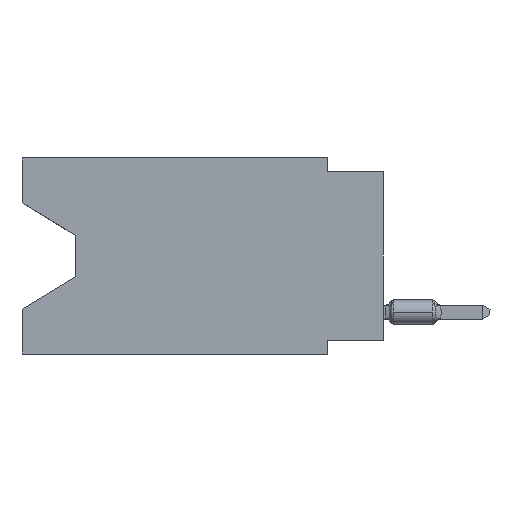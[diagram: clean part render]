
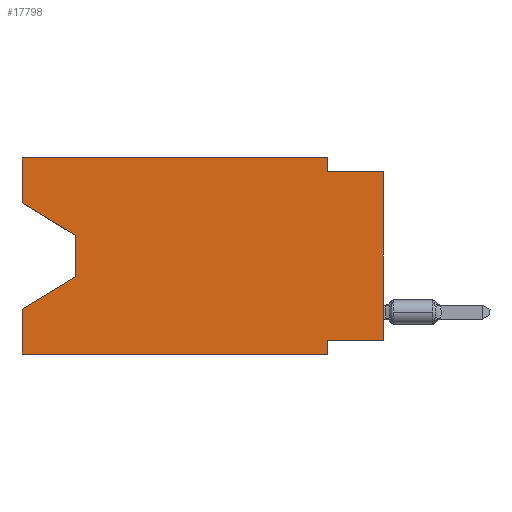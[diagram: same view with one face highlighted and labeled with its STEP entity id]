
A CAD part, left-side view. The second image highlights one B-rep face of the part: STEP entity #17798.
In plain terms, the highlighted planar face has unit normal (-1, 0, 0).
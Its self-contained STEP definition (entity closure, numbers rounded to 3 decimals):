
#36 = ORIENTED_EDGE ( 'NONE', *, *, #11473, .T. ) ;
#167 = VERTEX_POINT ( 'NONE', #1939 ) ;
#609 = DIRECTION ( 'NONE',  ( 0., 0., -1. ) ) ;
#623 = EDGE_LOOP ( 'NONE', ( #12350, #36, #3907, #7928, #14203, #6573, #1029, #13638, #10029, #7843, #1889, #755 ) ) ;
#755 = ORIENTED_EDGE ( 'NONE', *, *, #2708, .F. ) ;
#924 = CARTESIAN_POINT ( 'NONE',  ( 0., 0., -8.255 ) ) ;
#1029 = ORIENTED_EDGE ( 'NONE', *, *, #3658, .F. ) ;
#1125 = VECTOR ( 'NONE', #13891, 1000. ) ;
#1180 = EDGE_CURVE ( 'NONE', #12611, #2093, #13893, .T. ) ;
#1313 = LINE ( 'NONE', #5892, #17669 ) ;
#1889 = ORIENTED_EDGE ( 'NONE', *, *, #7205, .F. ) ;
#1939 = CARTESIAN_POINT ( 'NONE',  ( 0., 0., -8.255 ) ) ;
#2093 = VERTEX_POINT ( 'NONE', #7685 ) ;
#2153 = PLANE ( 'NONE',  #4093 ) ;
#2288 = EDGE_CURVE ( 'NONE', #17958, #12637, #5903, .T. ) ;
#2431 = CARTESIAN_POINT ( 'NONE',  ( 0., 2.54, -8.89 ) ) ;
#2708 = EDGE_CURVE ( 'NONE', #17958, #4142, #4644, .T. ) ;
#3041 = DIRECTION ( 'NONE',  ( 0., 0., -1. ) ) ;
#3259 = CARTESIAN_POINT ( 'NONE',  ( 0., 16.383, 0. ) ) ;
#3506 = VECTOR ( 'NONE', #12617, 1000. ) ;
#3658 = EDGE_CURVE ( 'NONE', #167, #11363, #8058, .T. ) ;
#3715 = CARTESIAN_POINT ( 'NONE',  ( 0., 13.97, -5.385 ) ) ;
#3753 = VERTEX_POINT ( 'NONE', #13911 ) ;
#3897 = CARTESIAN_POINT ( 'NONE',  ( 0., 13.97, -3.505 ) ) ;
#3907 = ORIENTED_EDGE ( 'NONE', *, *, #13072, .T. ) ;
#4093 = AXIS2_PLACEMENT_3D ( 'NONE', #7749, #14812, #609 ) ;
#4142 = VERTEX_POINT ( 'NONE', #12615 ) ;
#4143 = VERTEX_POINT ( 'NONE', #13811 ) ;
#4174 = EDGE_CURVE ( 'NONE', #13677, #12102, #8393, .T. ) ;
#4644 = LINE ( 'NONE', #10238, #10867 ) ;
#4886 = VECTOR ( 'NONE', #16300, 1000. ) ;
#5009 = CARTESIAN_POINT ( 'NONE',  ( 0., 16.383, -8.89 ) ) ;
#5292 = CARTESIAN_POINT ( 'NONE',  ( 0., 0., -0.635 ) ) ;
#5892 = CARTESIAN_POINT ( 'NONE',  ( 0., 2.54, 0. ) ) ;
#5903 = LINE ( 'NONE', #8487, #15532 ) ;
#5922 = CARTESIAN_POINT ( 'NONE',  ( 0., 2.54, -0.635 ) ) ;
#6031 = VECTOR ( 'NONE', #13901, 1000. ) ;
#6269 = EDGE_CURVE ( 'NONE', #3753, #13677, #1313, .T. ) ;
#6573 = ORIENTED_EDGE ( 'NONE', *, *, #12665, .F. ) ;
#7205 = EDGE_CURVE ( 'NONE', #4142, #3753, #17091, .T. ) ;
#7685 = CARTESIAN_POINT ( 'NONE',  ( 0., 2.54, -8.89 ) ) ;
#7749 = CARTESIAN_POINT ( 'NONE',  ( 0., 16.383, 0. ) ) ;
#7843 = ORIENTED_EDGE ( 'NONE', *, *, #6269, .F. ) ;
#7928 = ORIENTED_EDGE ( 'NONE', *, *, #16800, .F. ) ;
#8058 = LINE ( 'NONE', #924, #10163 ) ;
#8291 = DIRECTION ( 'NONE',  ( 0., 0., -1. ) ) ;
#8393 = LINE ( 'NONE', #5292, #1125 ) ;
#8407 = CARTESIAN_POINT ( 'NONE',  ( 0., 0., 0. ) ) ;
#8414 = VERTEX_POINT ( 'NONE', #3715 ) ;
#8487 = CARTESIAN_POINT ( 'NONE',  ( 0., 16.383, -2.038 ) ) ;
#8504 = LINE ( 'NONE', #8407, #6031 ) ;
#9122 = DIRECTION ( 'NONE',  ( 0., -1., 0. ) ) ;
#9284 = LINE ( 'NONE', #16158, #15175 ) ;
#9408 = CARTESIAN_POINT ( 'NONE',  ( 0., 13.97, -3.505 ) ) ;
#10029 = ORIENTED_EDGE ( 'NONE', *, *, #4174, .F. ) ;
#10070 = VECTOR ( 'NONE', #9122, 1000. ) ;
#10163 = VECTOR ( 'NONE', #14673, 1000. ) ;
#10238 = CARTESIAN_POINT ( 'NONE',  ( 0., 16.383, 0. ) ) ;
#10867 = VECTOR ( 'NONE', #13083, 1000. ) ;
#11222 = DIRECTION ( 'NONE',  ( 0., -0.855, -0.519 ) ) ;
#11363 = VERTEX_POINT ( 'NONE', #13539 ) ;
#11473 = EDGE_CURVE ( 'NONE', #12637, #8414, #12416, .T. ) ;
#12069 = FACE_OUTER_BOUND ( 'NONE', #623, .T. ) ;
#12102 = VERTEX_POINT ( 'NONE', #17488 ) ;
#12277 = CARTESIAN_POINT ( 'NONE',  ( 0., 16.383, 0. ) ) ;
#12350 = ORIENTED_EDGE ( 'NONE', *, *, #2288, .T. ) ;
#12416 = LINE ( 'NONE', #3897, #13729 ) ;
#12611 = VERTEX_POINT ( 'NONE', #5009 ) ;
#12615 = CARTESIAN_POINT ( 'NONE',  ( 0., 16.383, 0. ) ) ;
#12617 = DIRECTION ( 'NONE',  ( 0., -1., 0. ) ) ;
#12637 = VERTEX_POINT ( 'NONE', #9408 ) ;
#12665 = EDGE_CURVE ( 'NONE', #11363, #2093, #14999, .T. ) ;
#13072 = EDGE_CURVE ( 'NONE', #8414, #4143, #9284, .T. ) ;
#13083 = DIRECTION ( 'NONE',  ( 0., 0., 1. ) ) ;
#13539 = CARTESIAN_POINT ( 'NONE',  ( 0., 2.54, -8.255 ) ) ;
#13638 = ORIENTED_EDGE ( 'NONE', *, *, #15659, .T. ) ;
#13677 = VERTEX_POINT ( 'NONE', #5922 ) ;
#13729 = VECTOR ( 'NONE', #16717, 1000. ) ;
#13811 = CARTESIAN_POINT ( 'NONE',  ( 0., 16.383, -6.852 ) ) ;
#13891 = DIRECTION ( 'NONE',  ( 0., -1., 0. ) ) ;
#13893 = LINE ( 'NONE', #13993, #3506 ) ;
#13901 = DIRECTION ( 'NONE',  ( 0., 0., 1. ) ) ;
#13911 = CARTESIAN_POINT ( 'NONE',  ( 0., 2.54, 0. ) ) ;
#13993 = CARTESIAN_POINT ( 'NONE',  ( 0., 16.383, -8.89 ) ) ;
#14203 = ORIENTED_EDGE ( 'NONE', *, *, #1180, .T. ) ;
#14673 = DIRECTION ( 'NONE',  ( 0., 1., 0. ) ) ;
#14788 = DIRECTION ( 'NONE',  ( 0., 0.855, -0.519 ) ) ;
#14812 = DIRECTION ( 'NONE',  ( 1., 0., 0. ) ) ;
#14999 = LINE ( 'NONE', #2431, #16340 ) ;
#15175 = VECTOR ( 'NONE', #14788, 1000. ) ;
#15532 = VECTOR ( 'NONE', #11222, 1000. ) ;
#15659 = EDGE_CURVE ( 'NONE', #167, #12102, #8504, .T. ) ;
#16158 = CARTESIAN_POINT ( 'NONE',  ( 0., 13.97, -5.385 ) ) ;
#16300 = DIRECTION ( 'NONE',  ( 0., 0., 1. ) ) ;
#16340 = VECTOR ( 'NONE', #8291, 1000. ) ;
#16459 = CARTESIAN_POINT ( 'NONE',  ( 0., 16.383, -2.038 ) ) ;
#16565 = LINE ( 'NONE', #12277, #4886 ) ;
#16717 = DIRECTION ( 'NONE',  ( 0., 0., -1. ) ) ;
#16800 = EDGE_CURVE ( 'NONE', #12611, #4143, #16565, .T. ) ;
#17091 = LINE ( 'NONE', #3259, #10070 ) ;
#17488 = CARTESIAN_POINT ( 'NONE',  ( 0., 0., -0.635 ) ) ;
#17669 = VECTOR ( 'NONE', #3041, 1000. ) ;
#17798 = ADVANCED_FACE ( 'NONE', ( #12069 ), #2153, .F. ) ;
#17958 = VERTEX_POINT ( 'NONE', #16459 ) ;
